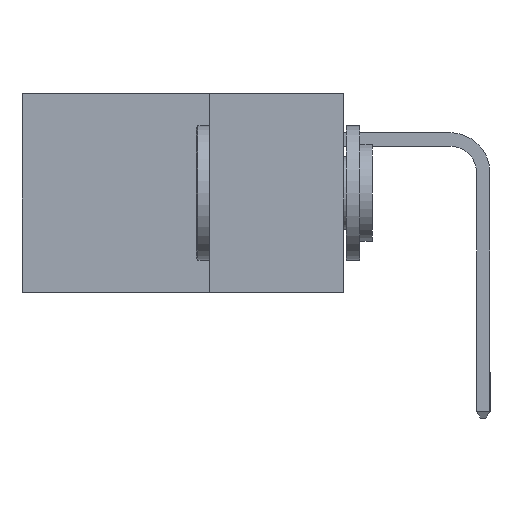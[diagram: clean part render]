
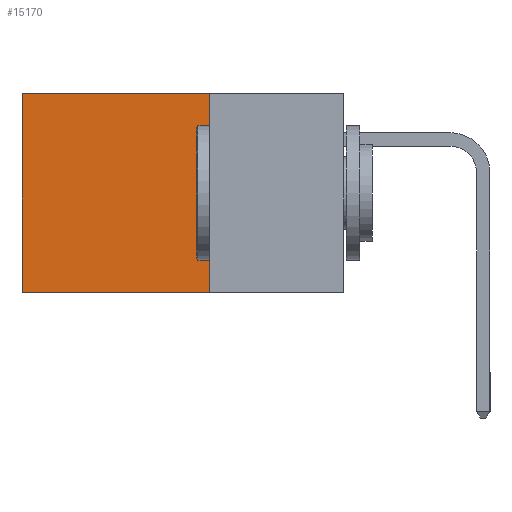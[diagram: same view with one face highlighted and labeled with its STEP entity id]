
A CAD part, left-side view. The second image highlights one B-rep face of the part: STEP entity #15170.
In plain terms, the highlighted planar face has unit normal (-1, 0, 0).
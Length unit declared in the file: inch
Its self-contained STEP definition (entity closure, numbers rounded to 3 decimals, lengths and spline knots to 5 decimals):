
#129 = EDGE_CURVE ( 'NONE', #9642, #8088, #14114, .T. ) ;
#343 = EDGE_LOOP ( 'NONE', ( #6600, #15077, #15674, #10183 ) ) ;
#461 = CARTESIAN_POINT ( 'NONE',  ( 0.2615, 0.25, 0. ) ) ;
#1282 = PLANE ( 'NONE',  #11870 ) ;
#1586 = LINE ( 'NONE', #5688, #15498 ) ;
#2357 = EDGE_CURVE ( 'NONE', #8088, #3354, #9427, .T. ) ;
#2437 = DIRECTION ( 'NONE',  ( 0., 0., -1. ) ) ;
#2627 = CARTESIAN_POINT ( 'NONE',  ( 0.2615, 0.25, 0. ) ) ;
#2952 = EDGE_CURVE ( 'NONE', #9642, #12701, #1586, .T. ) ;
#3354 = VERTEX_POINT ( 'NONE', #8074 ) ;
#4273 = EDGE_CURVE ( 'NONE', #12701, #3354, #14231, .T. ) ;
#5688 = CARTESIAN_POINT ( 'NONE',  ( 0.2615, 0.25, -0.37 ) ) ;
#6600 = ORIENTED_EDGE ( 'NONE', *, *, #2357, .T. ) ;
#6937 = DIRECTION ( 'NONE',  ( 0., 0., -1. ) ) ;
#8074 = CARTESIAN_POINT ( 'NONE',  ( 0.2615, 0.6, -0.37 ) ) ;
#8088 = VERTEX_POINT ( 'NONE', #11541 ) ;
#9416 = DIRECTION ( 'NONE',  ( 0., 0., -1. ) ) ;
#9427 = LINE ( 'NONE', #13308, #9691 ) ;
#9642 = VERTEX_POINT ( 'NONE', #2627 ) ;
#9691 = VECTOR ( 'NONE', #6937, 39.37008 ) ;
#9805 = DIRECTION ( 'NONE',  ( 1., 0., 0. ) ) ;
#10045 = CARTESIAN_POINT ( 'NONE',  ( 0.2615, 0.25, -0.37 ) ) ;
#10183 = ORIENTED_EDGE ( 'NONE', *, *, #129, .T. ) ;
#11541 = CARTESIAN_POINT ( 'NONE',  ( 0.2615, 0.6, 0. ) ) ;
#11870 = AXIS2_PLACEMENT_3D ( 'NONE', #13604, #9805, #2437 ) ;
#11906 = CARTESIAN_POINT ( 'NONE',  ( 0.2615, 0.25, -0.37 ) ) ;
#12701 = VERTEX_POINT ( 'NONE', #10045 ) ;
#13308 = CARTESIAN_POINT ( 'NONE',  ( 0.2615, 0.6, -0.37 ) ) ;
#13604 = CARTESIAN_POINT ( 'NONE',  ( 0.2615, 0.25, -0.37 ) ) ;
#14114 = LINE ( 'NONE', #461, #14468 ) ;
#14231 = LINE ( 'NONE', #11906, #15549 ) ;
#14337 = DIRECTION ( 'NONE',  ( 0., 1., 0. ) ) ;
#14468 = VECTOR ( 'NONE', #14337, 39.37008 ) ;
#14843 = FACE_OUTER_BOUND ( 'NONE', #343, .T. ) ;
#15077 = ORIENTED_EDGE ( 'NONE', *, *, #4273, .F. ) ;
#15170 = ADVANCED_FACE ( 'NONE', ( #14843 ), #1282, .F. ) ;
#15498 = VECTOR ( 'NONE', #9416, 39.37008 ) ;
#15549 = VECTOR ( 'NONE', #15698, 39.37008 ) ;
#15674 = ORIENTED_EDGE ( 'NONE', *, *, #2952, .F. ) ;
#15698 = DIRECTION ( 'NONE',  ( 0., 1., 0. ) ) ;
